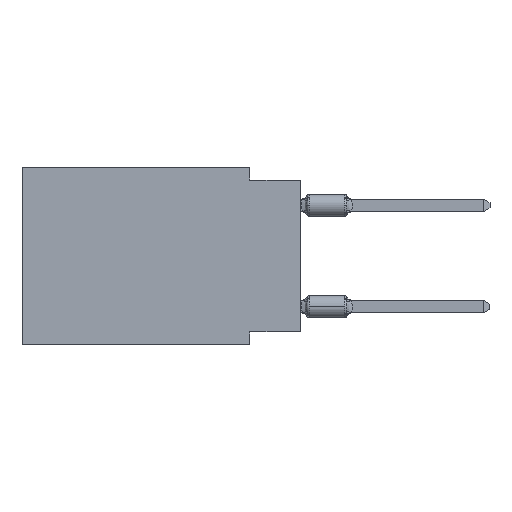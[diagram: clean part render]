
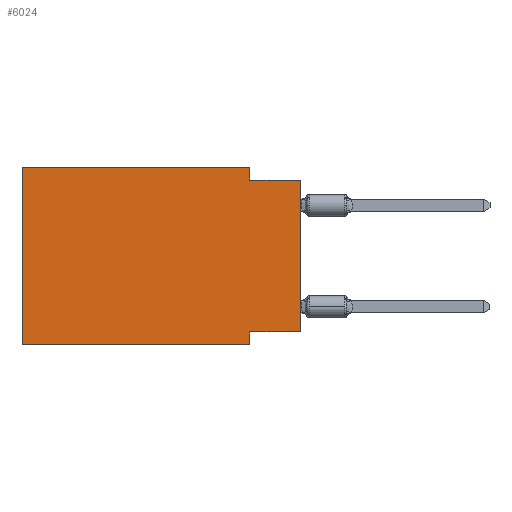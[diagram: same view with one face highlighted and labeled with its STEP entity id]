
A CAD part, left-side view. The second image highlights one B-rep face of the part: STEP entity #6024.
In plain terms, the highlighted planar face has unit normal (-1, 0, 0).
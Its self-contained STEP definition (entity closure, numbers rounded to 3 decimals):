
#223 = CARTESIAN_POINT ( 'NONE',  ( 0., 13.97, 0. ) ) ;
#246 = CARTESIAN_POINT ( 'NONE',  ( 0., 0., -8.255 ) ) ;
#255 = DIRECTION ( 'NONE',  ( 0., 0., -1. ) ) ;
#607 = CARTESIAN_POINT ( 'NONE',  ( 0., 0., -0.635 ) ) ;
#653 = CARTESIAN_POINT ( 'NONE',  ( 0., 2.54, 0. ) ) ;
#822 = EDGE_CURVE ( 'NONE', #2531, #1329, #10342, .T. ) ;
#1095 = VECTOR ( 'NONE', #5639, 1000. ) ;
#1292 = ORIENTED_EDGE ( 'NONE', *, *, #14624, .F. ) ;
#1329 = VERTEX_POINT ( 'NONE', #10331 ) ;
#1819 = CARTESIAN_POINT ( 'NONE',  ( 0., 2.54, -8.255 ) ) ;
#2201 = ORIENTED_EDGE ( 'NONE', *, *, #13806, .F. ) ;
#2234 = LINE ( 'NONE', #11267, #1095 ) ;
#2437 = CARTESIAN_POINT ( 'NONE',  ( 0., 2.54, -8.89 ) ) ;
#2531 = VERTEX_POINT ( 'NONE', #246 ) ;
#2574 = DIRECTION ( 'NONE',  ( 0., 0., -1. ) ) ;
#2775 = VERTEX_POINT ( 'NONE', #8566 ) ;
#3805 = DIRECTION ( 'NONE',  ( 1., 0., 0. ) ) ;
#3836 = ORIENTED_EDGE ( 'NONE', *, *, #9713, .F. ) ;
#3983 = AXIS2_PLACEMENT_3D ( 'NONE', #223, #3805, #2574 ) ;
#4226 = EDGE_CURVE ( 'NONE', #7611, #8832, #11461, .T. ) ;
#4502 = ORIENTED_EDGE ( 'NONE', *, *, #822, .T. ) ;
#4925 = CARTESIAN_POINT ( 'NONE',  ( 0., 13.97, 0. ) ) ;
#5023 = CARTESIAN_POINT ( 'NONE',  ( 0., 2.54, -0.635 ) ) ;
#5039 = PLANE ( 'NONE',  #3983 ) ;
#5047 = VERTEX_POINT ( 'NONE', #4925 ) ;
#5432 = LINE ( 'NONE', #10069, #12692 ) ;
#5639 = DIRECTION ( 'NONE',  ( 0., -1., 0. ) ) ;
#5655 = ORIENTED_EDGE ( 'NONE', *, *, #12881, .F. ) ;
#5787 = CARTESIAN_POINT ( 'NONE',  ( 0., 0., 0. ) ) ;
#5830 = DIRECTION ( 'NONE',  ( 0., 0., -1. ) ) ;
#6024 = ADVANCED_FACE ( 'NONE', ( #8454 ), #5039, .F. ) ;
#6638 = CARTESIAN_POINT ( 'NONE',  ( 0., 13.97, 0. ) ) ;
#6672 = CARTESIAN_POINT ( 'NONE',  ( 0., 2.54, -8.89 ) ) ;
#7000 = CARTESIAN_POINT ( 'NONE',  ( 0., 2.54, 0. ) ) ;
#7472 = LINE ( 'NONE', #607, #9698 ) ;
#7611 = VERTEX_POINT ( 'NONE', #1819 ) ;
#8454 = FACE_OUTER_BOUND ( 'NONE', #14058, .T. ) ;
#8566 = CARTESIAN_POINT ( 'NONE',  ( 0., 13.97, -8.89 ) ) ;
#8574 = ORIENTED_EDGE ( 'NONE', *, *, #12624, .T. ) ;
#8832 = VERTEX_POINT ( 'NONE', #6672 ) ;
#8948 = VECTOR ( 'NONE', #255, 1000. ) ;
#9698 = VECTOR ( 'NONE', #11121, 1000. ) ;
#9713 = EDGE_CURVE ( 'NONE', #5047, #10204, #12271, .T. ) ;
#9948 = VERTEX_POINT ( 'NONE', #5023 ) ;
#10069 = CARTESIAN_POINT ( 'NONE',  ( 0., 13.97, 0. ) ) ;
#10204 = VERTEX_POINT ( 'NONE', #653 ) ;
#10231 = ORIENTED_EDGE ( 'NONE', *, *, #15158, .F. ) ;
#10331 = CARTESIAN_POINT ( 'NONE',  ( 0., 0., -0.635 ) ) ;
#10342 = LINE ( 'NONE', #5787, #15044 ) ;
#10502 = CARTESIAN_POINT ( 'NONE',  ( 0., 0., -8.255 ) ) ;
#10604 = VECTOR ( 'NONE', #13564, 1000. ) ;
#10798 = ORIENTED_EDGE ( 'NONE', *, *, #4226, .F. ) ;
#11121 = DIRECTION ( 'NONE',  ( 0., -1., 0. ) ) ;
#11228 = VECTOR ( 'NONE', #5830, 1000. ) ;
#11267 = CARTESIAN_POINT ( 'NONE',  ( 0., 13.97, -8.89 ) ) ;
#11461 = LINE ( 'NONE', #2437, #11228 ) ;
#11706 = VECTOR ( 'NONE', #12718, 1000. ) ;
#11722 = LINE ( 'NONE', #7000, #8948 ) ;
#12271 = LINE ( 'NONE', #6638, #10604 ) ;
#12624 = EDGE_CURVE ( 'NONE', #2775, #8832, #2234, .T. ) ;
#12692 = VECTOR ( 'NONE', #13426, 1000. ) ;
#12710 = DIRECTION ( 'NONE',  ( 0., 0., 1. ) ) ;
#12718 = DIRECTION ( 'NONE',  ( 0., 1., 0. ) ) ;
#12797 = LINE ( 'NONE', #10502, #11706 ) ;
#12881 = EDGE_CURVE ( 'NONE', #10204, #9948, #11722, .T. ) ;
#13426 = DIRECTION ( 'NONE',  ( 0., 0., 1. ) ) ;
#13564 = DIRECTION ( 'NONE',  ( 0., -1., 0. ) ) ;
#13806 = EDGE_CURVE ( 'NONE', #9948, #1329, #7472, .T. ) ;
#14058 = EDGE_LOOP ( 'NONE', ( #4502, #2201, #5655, #3836, #10231, #8574, #10798, #1292 ) ) ;
#14624 = EDGE_CURVE ( 'NONE', #2531, #7611, #12797, .T. ) ;
#15044 = VECTOR ( 'NONE', #12710, 1000. ) ;
#15158 = EDGE_CURVE ( 'NONE', #2775, #5047, #5432, .T. ) ;
